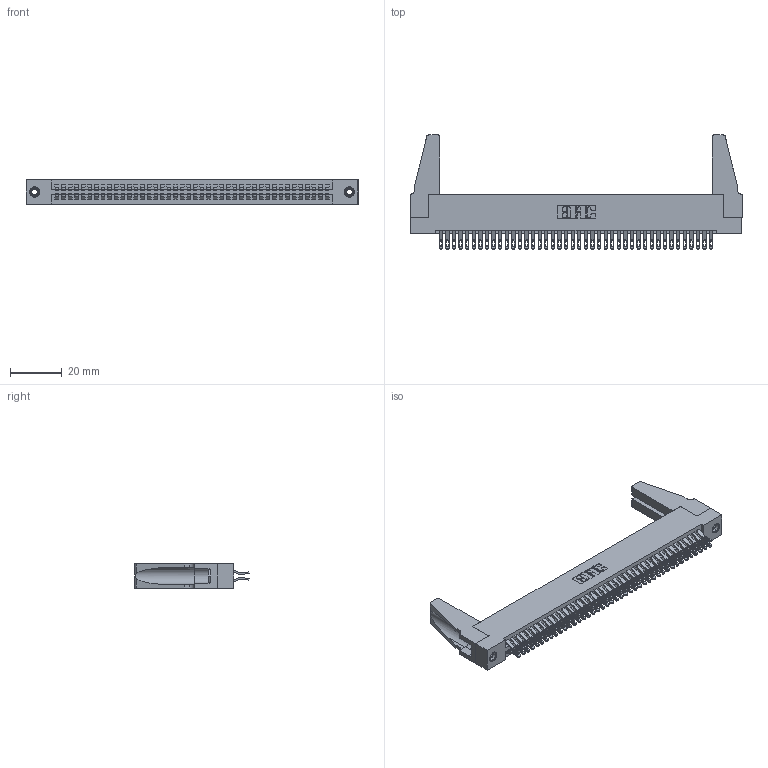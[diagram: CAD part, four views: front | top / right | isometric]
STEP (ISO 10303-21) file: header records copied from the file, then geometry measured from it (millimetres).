
FILE_DESCRIPTION (( 'STEP AP203' ), '1' );
FILE_NAME ('395-084-555-288.STEP', '2019-10-25T10:04:40', ( '' ), ( '' ), 'SwSTEP 2.0', 'SolidWorks 2016', '' );
FILE_SCHEMA (( 'CONFIG_CONTROL_DESIGN' ));
Length unit declared in the file: inch
Products named in the file (5): 345-250-001_345-250-001-102; 345-220-078_345-220-088; 395-084-555-288; 345 Part_Flush Mounting Lugs - 0.156 Dia-TH; 345-292-001_555 Tail
Assembly tree (89 placements, depth 2):
  395-084-555-288
    345 Part_Flush Mounting Lugs - 0.156 Dia-TH
    345-292-001_555 Tail  x84
    345-250-001_345-250-001-102  x2
    345-220-078_345-220-088  x2
Bounding box: 127.91 x 43.99 x 9.4 mm (x, y, z)
Volume: 15921.8 mm3; surface area: 22697 mm2
Topology: 89 solids, 89 shells, 4954 faces, 15523 edges, 10338 vertices
Faces by surface type: plane 2756, cylinder 2182, cone 12, torus 4
Entity records: 35428 total; most frequent: CARTESIAN_POINT 5968, ORIENTED_EDGE 5832, DIRECTION 5236, EDGE_CURVE 2916, VECTOR 2554, LINE 2554, VERTEX_POINT 1938, AXIS2_PLACEMENT_3D 1341
